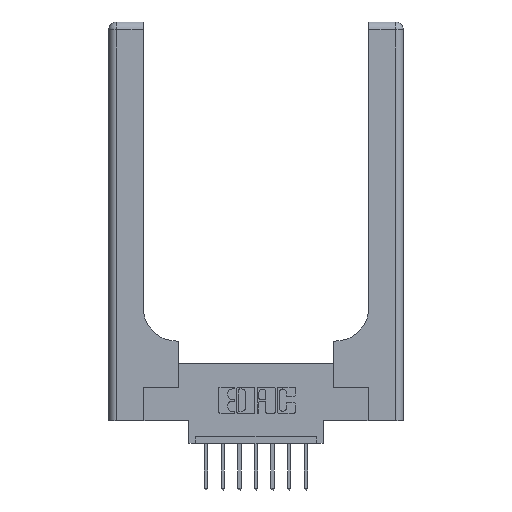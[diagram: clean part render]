
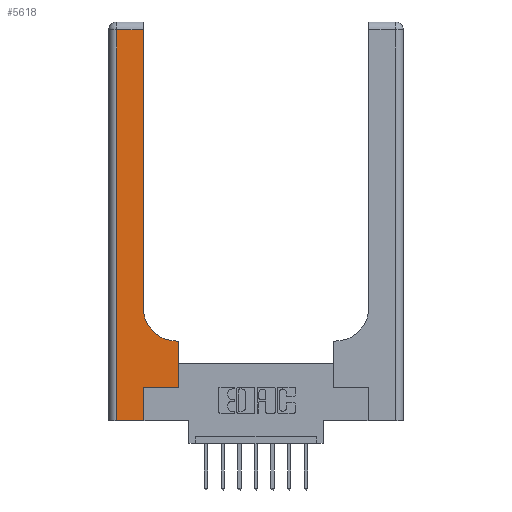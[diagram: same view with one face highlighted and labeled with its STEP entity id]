
A CAD part, top view. The second image highlights one B-rep face of the part: STEP entity #5618.
In plain terms, the highlighted planar face has unit normal (0, 0, 1).
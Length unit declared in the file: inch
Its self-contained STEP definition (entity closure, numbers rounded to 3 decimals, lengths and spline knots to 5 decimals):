
#32 = DIRECTION ( 'NONE',  ( 0., 0., -1. ) ) ;
#63 = DIRECTION ( 'NONE',  ( -1., 0., 0. ) ) ;
#73 = ORIENTED_EDGE ( 'NONE', *, *, #5848, .T. ) ;
#517 = CARTESIAN_POINT ( 'NONE',  ( 0.26, 0.85, 0.37 ) ) ;
#759 = DIRECTION ( 'NONE',  ( 1., 0., 0. ) ) ;
#1003 = VERTEX_POINT ( 'NONE', #14408 ) ;
#1190 = FACE_OUTER_BOUND ( 'NONE', #1219, .T. ) ;
#1219 = EDGE_LOOP ( 'NONE', ( #7156, #7927, #11993, #7908, #3071, #9980, #12122, #8560, #73 ) ) ;
#1410 = VECTOR ( 'NONE', #3096, 39.37008 ) ;
#1489 = VERTEX_POINT ( 'NONE', #5536 ) ;
#1798 = CARTESIAN_POINT ( 'NONE',  ( 0.26, 2.94, 0.37 ) ) ;
#1926 = CARTESIAN_POINT ( 'NONE',  ( 0.265, 0.25, 0.37 ) ) ;
#2218 = DIRECTION ( 'NONE',  ( -1., 0., 0. ) ) ;
#2498 = DIRECTION ( 'NONE',  ( -1., 0., 0. ) ) ;
#2692 = AXIS2_PLACEMENT_3D ( 'NONE', #5751, #10341, #63 ) ;
#3071 = ORIENTED_EDGE ( 'NONE', *, *, #14599, .T. ) ;
#3096 = DIRECTION ( 'NONE',  ( 0., 1., 0. ) ) ;
#3999 = VECTOR ( 'NONE', #9413, 39.37008 ) ;
#4116 = CARTESIAN_POINT ( 'NONE',  ( 0., 0., 0.37 ) ) ;
#4478 = VECTOR ( 'NONE', #5909, 39.37008 ) ;
#4557 = EDGE_CURVE ( 'NONE', #6496, #6733, #8198, .T. ) ;
#4624 = CIRCLE ( 'NONE', #14208, 0.25 ) ;
#4878 = LINE ( 'NONE', #4116, #7602 ) ;
#5179 = CARTESIAN_POINT ( 'NONE',  ( 0.265, 0., 0.37 ) ) ;
#5428 = VECTOR ( 'NONE', #2498, 39.37008 ) ;
#5535 = CARTESIAN_POINT ( 'NONE',  ( 0.06, 2.94, 0.37 ) ) ;
#5536 = CARTESIAN_POINT ( 'NONE',  ( 0.528, 0.6, 0.37 ) ) ;
#5618 = ADVANCED_FACE ( 'NONE', ( #1190 ), #12741, .F. ) ;
#5653 = LINE ( 'NONE', #7842, #8699 ) ;
#5751 = CARTESIAN_POINT ( 'NONE',  ( 0., 3., 0.37 ) ) ;
#5848 = EDGE_CURVE ( 'NONE', #1003, #6917, #4624, .T. ) ;
#5909 = DIRECTION ( 'NONE',  ( 0., -1., 0. ) ) ;
#6328 = DIRECTION ( 'NONE',  ( 1., 0., 0. ) ) ;
#6496 = VERTEX_POINT ( 'NONE', #1798 ) ;
#6497 = VERTEX_POINT ( 'NONE', #7279 ) ;
#6563 = CARTESIAN_POINT ( 'NONE',  ( 0.51, 0.85, 0.37 ) ) ;
#6733 = VERTEX_POINT ( 'NONE', #5535 ) ;
#6917 = VERTEX_POINT ( 'NONE', #517 ) ;
#7063 = EDGE_CURVE ( 'NONE', #10442, #6497, #13336, .T. ) ;
#7156 = ORIENTED_EDGE ( 'NONE', *, *, #13983, .T. ) ;
#7279 = CARTESIAN_POINT ( 'NONE',  ( 0.528, 0.25, 0.37 ) ) ;
#7598 = LINE ( 'NONE', #5179, #14316 ) ;
#7602 = VECTOR ( 'NONE', #759, 39.37008 ) ;
#7774 = EDGE_CURVE ( 'NONE', #10000, #11960, #4878, .T. ) ;
#7842 = CARTESIAN_POINT ( 'NONE',  ( 0.26, 0.6, 0.37 ) ) ;
#7908 = ORIENTED_EDGE ( 'NONE', *, *, #7774, .T. ) ;
#7927 = ORIENTED_EDGE ( 'NONE', *, *, #4557, .T. ) ;
#8125 = EDGE_CURVE ( 'NONE', #1489, #1003, #5653, .T. ) ;
#8198 = LINE ( 'NONE', #12792, #5428 ) ;
#8438 = LINE ( 'NONE', #8508, #3999 ) ;
#8462 = VECTOR ( 'NONE', #11172, 39.37008 ) ;
#8508 = CARTESIAN_POINT ( 'NONE',  ( 0.26, 3., 0.37 ) ) ;
#8560 = ORIENTED_EDGE ( 'NONE', *, *, #8125, .T. ) ;
#8699 = VECTOR ( 'NONE', #2218, 39.37008 ) ;
#8875 = DIRECTION ( 'NONE',  ( 0., 1., 0. ) ) ;
#9363 = EDGE_CURVE ( 'NONE', #6497, #1489, #14580, .T. ) ;
#9413 = DIRECTION ( 'NONE',  ( 0., 1., 0. ) ) ;
#9422 = CARTESIAN_POINT ( 'NONE',  ( 0.265, 0.25, 0.37 ) ) ;
#9980 = ORIENTED_EDGE ( 'NONE', *, *, #7063, .T. ) ;
#10000 = VERTEX_POINT ( 'NONE', #12397 ) ;
#10086 = CARTESIAN_POINT ( 'NONE',  ( 0.528, 0.25, 0.37 ) ) ;
#10139 = CARTESIAN_POINT ( 'NONE',  ( 0.265, 0., 0.37 ) ) ;
#10341 = DIRECTION ( 'NONE',  ( 0., 0., -1. ) ) ;
#10442 = VERTEX_POINT ( 'NONE', #9422 ) ;
#11172 = DIRECTION ( 'NONE',  ( 1., 0., 0. ) ) ;
#11960 = VERTEX_POINT ( 'NONE', #10139 ) ;
#11993 = ORIENTED_EDGE ( 'NONE', *, *, #13186, .T. ) ;
#12122 = ORIENTED_EDGE ( 'NONE', *, *, #9363, .T. ) ;
#12397 = CARTESIAN_POINT ( 'NONE',  ( 0.06, 0., 0.37 ) ) ;
#12697 = LINE ( 'NONE', #13887, #4478 ) ;
#12741 = PLANE ( 'NONE',  #2692 ) ;
#12792 = CARTESIAN_POINT ( 'NONE',  ( 0., 2.94, 0.37 ) ) ;
#13186 = EDGE_CURVE ( 'NONE', #6733, #10000, #12697, .T. ) ;
#13336 = LINE ( 'NONE', #1926, #8462 ) ;
#13887 = CARTESIAN_POINT ( 'NONE',  ( 0.06, 3., 0.37 ) ) ;
#13983 = EDGE_CURVE ( 'NONE', #6917, #6496, #8438, .T. ) ;
#14208 = AXIS2_PLACEMENT_3D ( 'NONE', #6563, #32, #6328 ) ;
#14316 = VECTOR ( 'NONE', #8875, 39.37008 ) ;
#14408 = CARTESIAN_POINT ( 'NONE',  ( 0.51, 0.6, 0.37 ) ) ;
#14580 = LINE ( 'NONE', #10086, #1410 ) ;
#14599 = EDGE_CURVE ( 'NONE', #11960, #10442, #7598, .T. ) ;
